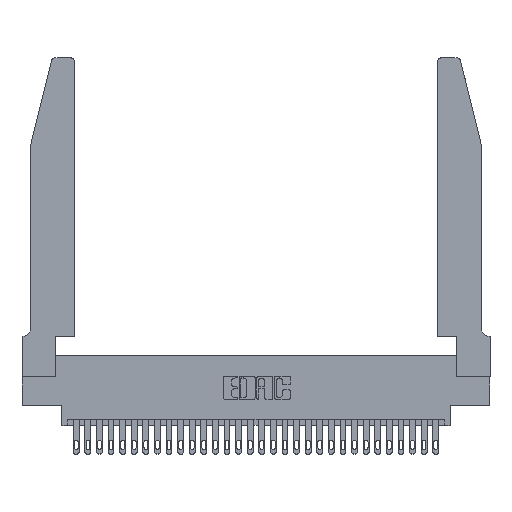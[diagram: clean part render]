
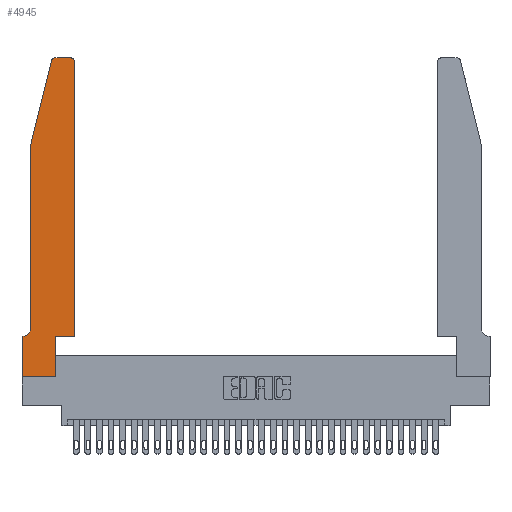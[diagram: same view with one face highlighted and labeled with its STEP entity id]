
A CAD part, top view. The second image highlights one B-rep face of the part: STEP entity #4945.
In plain terms, the highlighted planar face has unit normal (0, 0, 1).
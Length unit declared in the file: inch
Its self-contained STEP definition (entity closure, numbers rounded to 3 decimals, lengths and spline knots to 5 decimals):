
#93 = CARTESIAN_POINT ( 'NONE',  ( 0.0755, 0.42, 0.37 ) ) ;
#127 = LINE ( 'NONE', #6507, #25025 ) ;
#263 = DIRECTION ( 'NONE',  ( 0., 0., -1. ) ) ;
#1021 = VECTOR ( 'NONE', #28869, 39.37008 ) ;
#1027 = ORIENTED_EDGE ( 'NONE', *, *, #14602, .T. ) ;
#1262 = LINE ( 'NONE', #28320, #19782 ) ;
#1387 = CIRCLE ( 'NONE', #30217, 0.07 ) ;
#1426 = EDGE_CURVE ( 'NONE', #23120, #21649, #1387, .T. ) ;
#1500 = ORIENTED_EDGE ( 'NONE', *, *, #3955, .T. ) ;
#1544 = CARTESIAN_POINT ( 'NONE',  ( 0.0755, 2., 0.37 ) ) ;
#1553 = LINE ( 'NONE', #19961, #23104 ) ;
#1635 = CARTESIAN_POINT ( 'NONE',  ( 0.4205, 2.72, 0.37 ) ) ;
#1716 = DIRECTION ( 'NONE',  ( -1., 0., 0. ) ) ;
#1813 = PLANE ( 'NONE',  #11367 ) ;
#1973 = CARTESIAN_POINT ( 'NONE',  ( 0.284, 2.72, 0.37 ) ) ;
#2420 = ORIENTED_EDGE ( 'NONE', *, *, #26349, .T. ) ;
#2480 = VERTEX_POINT ( 'NONE', #28269 ) ;
#3216 = LINE ( 'NONE', #20213, #15688 ) ;
#3248 = CIRCLE ( 'NONE', #18858, 0.03 ) ;
#3713 = DIRECTION ( 'NONE',  ( 0., 1., 0. ) ) ;
#3744 = CARTESIAN_POINT ( 'NONE',  ( 0., 0.35, 0.37 ) ) ;
#3955 = EDGE_CURVE ( 'NONE', #18902, #2480, #21880, .T. ) ;
#4450 = CARTESIAN_POINT ( 'NONE',  ( 0., 0.35, 0.37 ) ) ;
#4492 = CARTESIAN_POINT ( 'NONE',  ( 0., 0., 0.37 ) ) ;
#4820 = ORIENTED_EDGE ( 'NONE', *, *, #5131, .T. ) ;
#4945 = ADVANCED_FACE ( 'NONE', ( #12739 ), #1813, .T. ) ;
#5131 = EDGE_CURVE ( 'NONE', #12213, #17383, #21830, .T. ) ;
#6290 = CARTESIAN_POINT ( 'NONE',  ( 0.284, 2.75, 0.37 ) ) ;
#6483 = CARTESIAN_POINT ( 'NONE',  ( 0.2605, 2.75, 0.37 ) ) ;
#6507 = CARTESIAN_POINT ( 'NONE',  ( 0.4505, 0.35, 0.37 ) ) ;
#6740 = DIRECTION ( 'NONE',  ( 0., 0., 1. ) ) ;
#6819 = DIRECTION ( 'NONE',  ( 0., 0., 1. ) ) ;
#7005 = CIRCLE ( 'NONE', #26539, 0.03 ) ;
#7124 = VERTEX_POINT ( 'NONE', #20469 ) ;
#9340 = DIRECTION ( 'NONE',  ( 0., 1., 0. ) ) ;
#9925 = VECTOR ( 'NONE', #3713, 39.37008 ) ;
#10096 = EDGE_CURVE ( 'NONE', #7124, #12213, #18614, .T. ) ;
#11347 = VERTEX_POINT ( 'NONE', #6290 ) ;
#11367 = AXIS2_PLACEMENT_3D ( 'NONE', #4450, #19029, #21252 ) ;
#11964 = VERTEX_POINT ( 'NONE', #30121 ) ;
#11982 = DIRECTION ( 'NONE',  ( 1., 0., 0. ) ) ;
#12213 = VERTEX_POINT ( 'NONE', #14134 ) ;
#12222 = ORIENTED_EDGE ( 'NONE', *, *, #21973, .T. ) ;
#12722 = ORIENTED_EDGE ( 'NONE', *, *, #14462, .T. ) ;
#12739 = FACE_OUTER_BOUND ( 'NONE', #13077, .T. ) ;
#13077 = EDGE_LOOP ( 'NONE', ( #18421, #23627, #1500, #12722, #28509, #23511, #12222, #2420, #13216, #4820, #19021, #1027 ) ) ;
#13216 = ORIENTED_EDGE ( 'NONE', *, *, #10096, .T. ) ;
#13339 = CARTESIAN_POINT ( 'NONE',  ( 0.2865, 0.35, 0.37 ) ) ;
#13451 = DIRECTION ( 'NONE',  ( -1., 0., 0. ) ) ;
#13713 = CARTESIAN_POINT ( 'NONE',  ( 0., 0., 0.37 ) ) ;
#13885 = VERTEX_POINT ( 'NONE', #13713 ) ;
#14134 = CARTESIAN_POINT ( 'NONE',  ( 0.2865, 0.35, 0.37 ) ) ;
#14330 = DIRECTION ( 'NONE',  ( 1., 0., 0. ) ) ;
#14419 = VECTOR ( 'NONE', #13451, 39.37008 ) ;
#14462 = EDGE_CURVE ( 'NONE', #2480, #23120, #3216, .T. ) ;
#14602 = EDGE_CURVE ( 'NONE', #27623, #11964, #7005, .T. ) ;
#14898 = LINE ( 'NONE', #4492, #19424 ) ;
#15688 = VECTOR ( 'NONE', #25408, 39.37008 ) ;
#16034 = CARTESIAN_POINT ( 'NONE',  ( 0.25487, 2.72718, 0.37 ) ) ;
#16148 = DIRECTION ( 'NONE',  ( -0.239, -0.971, 0. ) ) ;
#16421 = CARTESIAN_POINT ( 'NONE',  ( 0.0055, 0.35, 0.37 ) ) ;
#17148 = DIRECTION ( 'NONE',  ( -1., 0., 0. ) ) ;
#17383 = VERTEX_POINT ( 'NONE', #30178 ) ;
#17666 = EDGE_CURVE ( 'NONE', #11347, #18902, #3248, .T. ) ;
#18421 = ORIENTED_EDGE ( 'NONE', *, *, #30695, .T. ) ;
#18614 = LINE ( 'NONE', #13339, #9925 ) ;
#18858 = AXIS2_PLACEMENT_3D ( 'NONE', #1973, #6740, #18971 ) ;
#18902 = VERTEX_POINT ( 'NONE', #16034 ) ;
#18971 = DIRECTION ( 'NONE',  ( 1., 0., 0. ) ) ;
#19021 = ORIENTED_EDGE ( 'NONE', *, *, #27565, .T. ) ;
#19029 = DIRECTION ( 'NONE',  ( 0., 0., 1. ) ) ;
#19238 = CARTESIAN_POINT ( 'NONE',  ( 0.4505, 0.35, 0.37 ) ) ;
#19424 = VECTOR ( 'NONE', #14330, 39.37008 ) ;
#19782 = VECTOR ( 'NONE', #1716, 39.37008 ) ;
#19961 = CARTESIAN_POINT ( 'NONE',  ( 0., 0., 0.37 ) ) ;
#20213 = CARTESIAN_POINT ( 'NONE',  ( 0.0755, 2., 0.37 ) ) ;
#20264 = DIRECTION ( 'NONE',  ( 0., -1., 0. ) ) ;
#20469 = CARTESIAN_POINT ( 'NONE',  ( 0.2865, 0., 0.37 ) ) ;
#20779 = VERTEX_POINT ( 'NONE', #3744 ) ;
#21252 = DIRECTION ( 'NONE',  ( 1., 0., 0. ) ) ;
#21649 = VERTEX_POINT ( 'NONE', #16421 ) ;
#21830 = LINE ( 'NONE', #19238, #1021 ) ;
#21880 = LINE ( 'NONE', #1544, #27170 ) ;
#21973 = EDGE_CURVE ( 'NONE', #20779, #13885, #1553, .T. ) ;
#23104 = VECTOR ( 'NONE', #20264, 39.37008 ) ;
#23120 = VERTEX_POINT ( 'NONE', #93 ) ;
#23511 = ORIENTED_EDGE ( 'NONE', *, *, #26914, .T. ) ;
#23627 = ORIENTED_EDGE ( 'NONE', *, *, #17666, .T. ) ;
#25025 = VECTOR ( 'NONE', #9340, 39.37008 ) ;
#25408 = DIRECTION ( 'NONE',  ( 0., -1., 0. ) ) ;
#26349 = EDGE_CURVE ( 'NONE', #13885, #7124, #14898, .T. ) ;
#26525 = LINE ( 'NONE', #6483, #14419 ) ;
#26539 = AXIS2_PLACEMENT_3D ( 'NONE', #1635, #6819, #11982 ) ;
#26914 = EDGE_CURVE ( 'NONE', #21649, #20779, #1262, .T. ) ;
#27170 = VECTOR ( 'NONE', #16148, 39.37008 ) ;
#27565 = EDGE_CURVE ( 'NONE', #17383, #27623, #127, .T. ) ;
#27623 = VERTEX_POINT ( 'NONE', #30905 ) ;
#28269 = CARTESIAN_POINT ( 'NONE',  ( 0.0755, 2., 0.37 ) ) ;
#28320 = CARTESIAN_POINT ( 'NONE',  ( 0.0755, 0.35, 0.37 ) ) ;
#28509 = ORIENTED_EDGE ( 'NONE', *, *, #1426, .T. ) ;
#28869 = DIRECTION ( 'NONE',  ( 1., 0., 0. ) ) ;
#29698 = CARTESIAN_POINT ( 'NONE',  ( 0.0055, 0.42, 0.37 ) ) ;
#30121 = CARTESIAN_POINT ( 'NONE',  ( 0.4205, 2.75, 0.37 ) ) ;
#30178 = CARTESIAN_POINT ( 'NONE',  ( 0.4505, 0.35, 0.37 ) ) ;
#30217 = AXIS2_PLACEMENT_3D ( 'NONE', #29698, #263, #17148 ) ;
#30695 = EDGE_CURVE ( 'NONE', #11964, #11347, #26525, .T. ) ;
#30905 = CARTESIAN_POINT ( 'NONE',  ( 0.4505, 2.72, 0.37 ) ) ;
